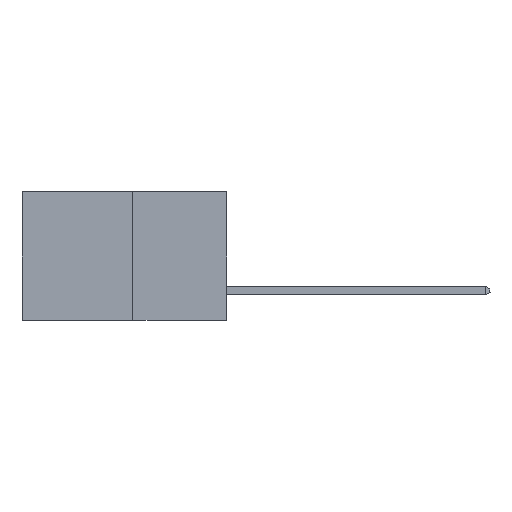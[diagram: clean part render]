
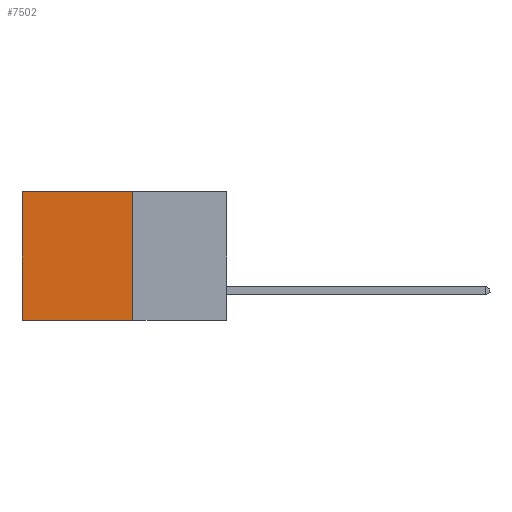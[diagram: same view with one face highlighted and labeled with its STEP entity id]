
A CAD part, left-side view. The second image highlights one B-rep face of the part: STEP entity #7502.
In plain terms, the highlighted planar face has unit normal (-1, 0, 0).
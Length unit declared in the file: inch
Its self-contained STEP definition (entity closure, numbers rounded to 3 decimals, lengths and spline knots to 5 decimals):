
#436 = DIRECTION ( 'NONE',  ( 0., 1., 0. ) ) ;
#527 = EDGE_CURVE ( 'NONE', #5889, #8515, #9249, .T. ) ;
#721 = DIRECTION ( 'NONE',  ( 1., 0., 0. ) ) ;
#772 = VECTOR ( 'NONE', #11812, 39.37008 ) ;
#1215 = ORIENTED_EDGE ( 'NONE', *, *, #527, .T. ) ;
#1425 = EDGE_CURVE ( 'NONE', #9199, #8515, #8646, .T. ) ;
#1758 = PLANE ( 'NONE',  #12408 ) ;
#2676 = CARTESIAN_POINT ( 'NONE',  ( 0.277, 0.27, 0. ) ) ;
#4124 = VERTEX_POINT ( 'NONE', #2676 ) ;
#4126 = VECTOR ( 'NONE', #6063, 39.37008 ) ;
#4164 = EDGE_CURVE ( 'NONE', #4124, #9199, #5594, .T. ) ;
#4174 = CARTESIAN_POINT ( 'NONE',  ( 0.277, 0.59, -0.37 ) ) ;
#5594 = LINE ( 'NONE', #12181, #10088 ) ;
#5718 = LINE ( 'NONE', #7389, #8003 ) ;
#5889 = VERTEX_POINT ( 'NONE', #9461 ) ;
#5947 = EDGE_LOOP ( 'NONE', ( #1215, #6501, #9032, #11465 ) ) ;
#6063 = DIRECTION ( 'NONE',  ( 0., 0., -1. ) ) ;
#6176 = CARTESIAN_POINT ( 'NONE',  ( 0.277, 0.59, -0.37 ) ) ;
#6348 = CARTESIAN_POINT ( 'NONE',  ( 0.277, 0.27, -0.37 ) ) ;
#6501 = ORIENTED_EDGE ( 'NONE', *, *, #1425, .F. ) ;
#6696 = CARTESIAN_POINT ( 'NONE',  ( 0.277, 0.27, -0.37 ) ) ;
#7389 = CARTESIAN_POINT ( 'NONE',  ( 0.277, 0.27, 0. ) ) ;
#7502 = ADVANCED_FACE ( 'NONE', ( #11070 ), #1758, .F. ) ;
#7659 = DIRECTION ( 'NONE',  ( 0., 0., -1. ) ) ;
#8003 = VECTOR ( 'NONE', #436, 39.37008 ) ;
#8014 = EDGE_CURVE ( 'NONE', #4124, #5889, #5718, .T. ) ;
#8515 = VERTEX_POINT ( 'NONE', #6176 ) ;
#8646 = LINE ( 'NONE', #6348, #772 ) ;
#9032 = ORIENTED_EDGE ( 'NONE', *, *, #4164, .F. ) ;
#9199 = VERTEX_POINT ( 'NONE', #12565 ) ;
#9249 = LINE ( 'NONE', #4174, #4126 ) ;
#9461 = CARTESIAN_POINT ( 'NONE',  ( 0.277, 0.59, 0. ) ) ;
#10088 = VECTOR ( 'NONE', #12239, 39.37008 ) ;
#11070 = FACE_OUTER_BOUND ( 'NONE', #5947, .T. ) ;
#11465 = ORIENTED_EDGE ( 'NONE', *, *, #8014, .T. ) ;
#11812 = DIRECTION ( 'NONE',  ( 0., 1., 0. ) ) ;
#12181 = CARTESIAN_POINT ( 'NONE',  ( 0.277, 0.27, -0.37 ) ) ;
#12239 = DIRECTION ( 'NONE',  ( 0., 0., -1. ) ) ;
#12408 = AXIS2_PLACEMENT_3D ( 'NONE', #6696, #721, #7659 ) ;
#12565 = CARTESIAN_POINT ( 'NONE',  ( 0.277, 0.27, -0.37 ) ) ;
